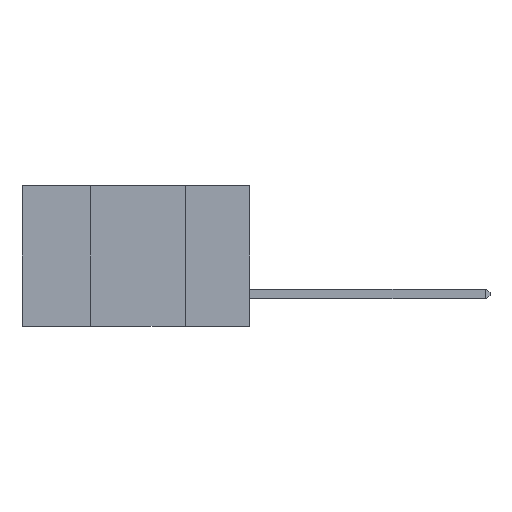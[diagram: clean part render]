
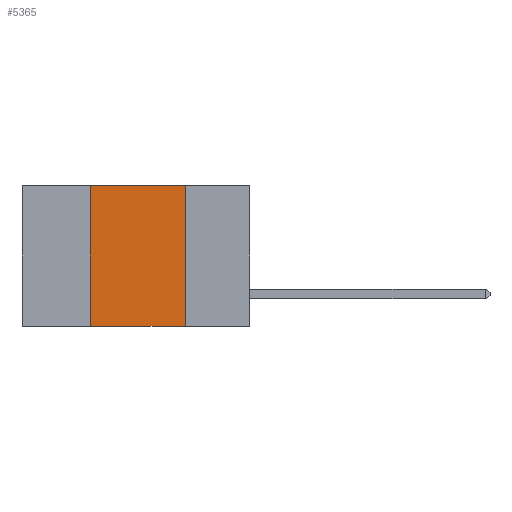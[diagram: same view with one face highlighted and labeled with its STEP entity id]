
A CAD part, left-side view. The second image highlights one B-rep face of the part: STEP entity #5365.
In plain terms, the highlighted planar face has unit normal (-1, 0, 0).
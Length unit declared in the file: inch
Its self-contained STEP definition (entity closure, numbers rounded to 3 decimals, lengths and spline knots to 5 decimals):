
#282 = EDGE_CURVE ( 'NONE', #3420, #5342, #4117, .T. ) ;
#490 = DIRECTION ( 'NONE',  ( 1., 0., 0. ) ) ;
#769 = EDGE_CURVE ( 'NONE', #1775, #3420, #7351, .T. ) ;
#1255 = CARTESIAN_POINT ( 'NONE',  ( 0., 0.42, -0.37 ) ) ;
#1396 = VERTEX_POINT ( 'NONE', #2341 ) ;
#1486 = VECTOR ( 'NONE', #7891, 39.37008 ) ;
#1678 = AXIS2_PLACEMENT_3D ( 'NONE', #8305, #490, #7395 ) ;
#1722 = ORIENTED_EDGE ( 'NONE', *, *, #11876, .F. ) ;
#1775 = VERTEX_POINT ( 'NONE', #1255 ) ;
#1821 = ORIENTED_EDGE ( 'NONE', *, *, #282, .F. ) ;
#1878 = ORIENTED_EDGE ( 'NONE', *, *, #769, .F. ) ;
#1910 = ORIENTED_EDGE ( 'NONE', *, *, #10475, .T. ) ;
#2341 = CARTESIAN_POINT ( 'NONE',  ( 0., 0.17, -0.37 ) ) ;
#3420 = VERTEX_POINT ( 'NONE', #10681 ) ;
#3916 = EDGE_LOOP ( 'NONE', ( #1722, #1821, #1878, #1910 ) ) ;
#4117 = LINE ( 'NONE', #5757, #1486 ) ;
#4990 = CARTESIAN_POINT ( 'NONE',  ( 0., 0.17, 0. ) ) ;
#5342 = VERTEX_POINT ( 'NONE', #11902 ) ;
#5365 = ADVANCED_FACE ( 'NONE', ( #5954 ), #11943, .F. ) ;
#5757 = CARTESIAN_POINT ( 'NONE',  ( 0., 0.6, 0. ) ) ;
#5954 = FACE_OUTER_BOUND ( 'NONE', #3916, .T. ) ;
#6247 = VECTOR ( 'NONE', #12299, 39.37008 ) ;
#6827 = CARTESIAN_POINT ( 'NONE',  ( 0., 0.6, -0.37 ) ) ;
#7351 = LINE ( 'NONE', #11793, #7644 ) ;
#7395 = DIRECTION ( 'NONE',  ( 0., 0., -1. ) ) ;
#7644 = VECTOR ( 'NONE', #11820, 39.37008 ) ;
#7891 = DIRECTION ( 'NONE',  ( 0., -1., 0. ) ) ;
#7926 = DIRECTION ( 'NONE',  ( 0., 0., -1. ) ) ;
#8305 = CARTESIAN_POINT ( 'NONE',  ( 0., 0.6, 0. ) ) ;
#9755 = LINE ( 'NONE', #4990, #11852 ) ;
#10475 = EDGE_CURVE ( 'NONE', #1775, #1396, #11192, .T. ) ;
#10681 = CARTESIAN_POINT ( 'NONE',  ( 0., 0.42, 0. ) ) ;
#11192 = LINE ( 'NONE', #6827, #6247 ) ;
#11793 = CARTESIAN_POINT ( 'NONE',  ( 0., 0.42, 0. ) ) ;
#11820 = DIRECTION ( 'NONE',  ( 0., 0., 1. ) ) ;
#11852 = VECTOR ( 'NONE', #7926, 39.37008 ) ;
#11876 = EDGE_CURVE ( 'NONE', #5342, #1396, #9755, .T. ) ;
#11902 = CARTESIAN_POINT ( 'NONE',  ( 0., 0.17, 0. ) ) ;
#11943 = PLANE ( 'NONE',  #1678 ) ;
#12299 = DIRECTION ( 'NONE',  ( 0., -1., 0. ) ) ;
